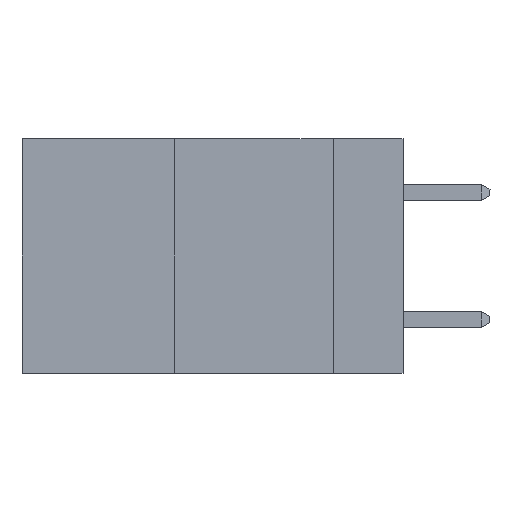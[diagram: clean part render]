
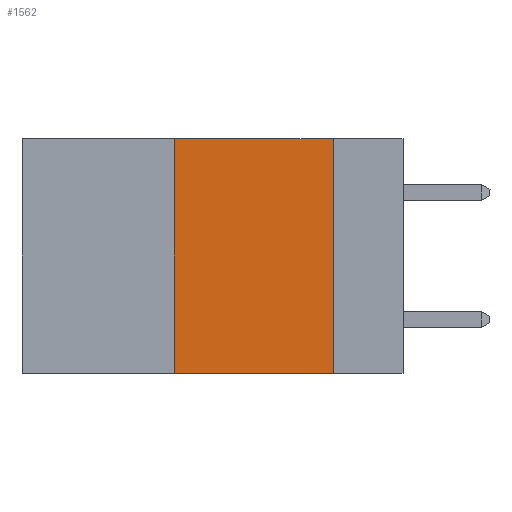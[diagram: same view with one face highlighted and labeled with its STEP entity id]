
A CAD part, left-side view. The second image highlights one B-rep face of the part: STEP entity #1562.
In plain terms, the highlighted planar face has unit normal (-1, 0, 0).
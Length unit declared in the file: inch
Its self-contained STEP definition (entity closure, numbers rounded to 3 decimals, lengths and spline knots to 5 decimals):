
#388 = VERTEX_POINT ( 'NONE', #562 ) ;
#562 = CARTESIAN_POINT ( 'NONE',  ( 0., 0.36, 0. ) ) ;
#573 = ORIENTED_EDGE ( 'NONE', *, *, #8052, .T. ) ;
#878 = LINE ( 'NONE', #9871, #5891 ) ;
#1349 = VECTOR ( 'NONE', #7869, 39.37008 ) ;
#1562 = ADVANCED_FACE ( 'NONE', ( #7834 ), #7201, .F. ) ;
#1565 = EDGE_CURVE ( 'NONE', #1960, #388, #10282, .T. ) ;
#1960 = VERTEX_POINT ( 'NONE', #2543 ) ;
#2150 = LINE ( 'NONE', #9270, #7341 ) ;
#2297 = VERTEX_POINT ( 'NONE', #4619 ) ;
#2543 = CARTESIAN_POINT ( 'NONE',  ( 0., 0.36, -0.37 ) ) ;
#3162 = ORIENTED_EDGE ( 'NONE', *, *, #6528, .F. ) ;
#4030 = DIRECTION ( 'NONE',  ( 0., 0., -1. ) ) ;
#4214 = EDGE_CURVE ( 'NONE', #388, #2297, #2150, .T. ) ;
#4219 = LINE ( 'NONE', #12433, #1349 ) ;
#4619 = CARTESIAN_POINT ( 'NONE',  ( 0., 0.11, 0. ) ) ;
#5190 = VECTOR ( 'NONE', #7031, 39.37008 ) ;
#5891 = VECTOR ( 'NONE', #4030, 39.37008 ) ;
#5946 = ORIENTED_EDGE ( 'NONE', *, *, #4214, .F. ) ;
#6215 = EDGE_LOOP ( 'NONE', ( #3162, #5946, #8497, #573 ) ) ;
#6499 = DIRECTION ( 'NONE',  ( 0., -1., 0. ) ) ;
#6528 = EDGE_CURVE ( 'NONE', #2297, #10956, #878, .T. ) ;
#6781 = CARTESIAN_POINT ( 'NONE',  ( 0., 0.36, 0. ) ) ;
#6860 = DIRECTION ( 'NONE',  ( 0., 0., -1. ) ) ;
#6873 = DIRECTION ( 'NONE',  ( 1., 0., 0. ) ) ;
#6876 = CARTESIAN_POINT ( 'NONE',  ( 0., 0.6, 0. ) ) ;
#7031 = DIRECTION ( 'NONE',  ( 0., 0., 1. ) ) ;
#7054 = CARTESIAN_POINT ( 'NONE',  ( 0., 0.11, -0.37 ) ) ;
#7171 = AXIS2_PLACEMENT_3D ( 'NONE', #6876, #6873, #6860 ) ;
#7201 = PLANE ( 'NONE',  #7171 ) ;
#7341 = VECTOR ( 'NONE', #6499, 39.37008 ) ;
#7834 = FACE_OUTER_BOUND ( 'NONE', #6215, .T. ) ;
#7869 = DIRECTION ( 'NONE',  ( 0., -1., 0. ) ) ;
#8052 = EDGE_CURVE ( 'NONE', #1960, #10956, #4219, .T. ) ;
#8497 = ORIENTED_EDGE ( 'NONE', *, *, #1565, .F. ) ;
#9270 = CARTESIAN_POINT ( 'NONE',  ( 0., 0.6, 0. ) ) ;
#9871 = CARTESIAN_POINT ( 'NONE',  ( 0., 0.11, 0. ) ) ;
#10282 = LINE ( 'NONE', #6781, #5190 ) ;
#10956 = VERTEX_POINT ( 'NONE', #7054 ) ;
#12433 = CARTESIAN_POINT ( 'NONE',  ( 0., 0.6, -0.37 ) ) ;
